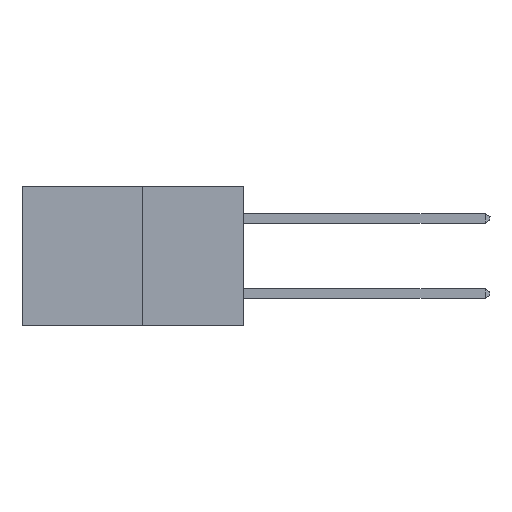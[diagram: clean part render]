
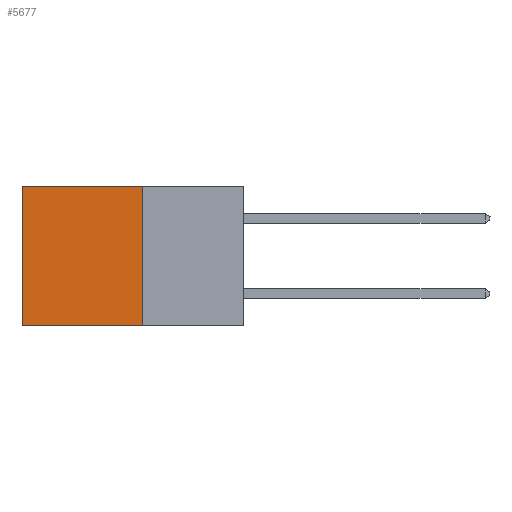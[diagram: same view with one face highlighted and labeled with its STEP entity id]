
A CAD part, left-side view. The second image highlights one B-rep face of the part: STEP entity #5677.
In plain terms, the highlighted planar face has unit normal (-1, 0, 0).
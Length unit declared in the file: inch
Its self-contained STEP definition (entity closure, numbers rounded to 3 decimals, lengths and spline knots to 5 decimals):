
#43 = ORIENTED_EDGE ( 'NONE', *, *, #1094, .T. ) ;
#718 = ORIENTED_EDGE ( 'NONE', *, *, #7204, .F. ) ;
#1094 = EDGE_CURVE ( 'NONE', #8426, #3668, #2150, .T. ) ;
#1461 = EDGE_CURVE ( 'NONE', #3668, #2317, #6913, .T. ) ;
#1546 = VECTOR ( 'NONE', #2091, 39.37008 ) ;
#1614 = CARTESIAN_POINT ( 'NONE',  ( 0.277, 0.27, -0.37 ) ) ;
#1648 = DIRECTION ( 'NONE',  ( 0., 1., 0. ) ) ;
#1667 = ORIENTED_EDGE ( 'NONE', *, *, #1461, .T. ) ;
#1909 = ORIENTED_EDGE ( 'NONE', *, *, #2686, .F. ) ;
#2091 = DIRECTION ( 'NONE',  ( 0., 1., 0. ) ) ;
#2150 = LINE ( 'NONE', #7919, #7536 ) ;
#2317 = VERTEX_POINT ( 'NONE', #6394 ) ;
#2346 = VERTEX_POINT ( 'NONE', #6817 ) ;
#2375 = DIRECTION ( 'NONE',  ( 0., 0., -1. ) ) ;
#2686 = EDGE_CURVE ( 'NONE', #2346, #2317, #3247, .T. ) ;
#2701 = FACE_OUTER_BOUND ( 'NONE', #6406, .T. ) ;
#3247 = LINE ( 'NONE', #8057, #1546 ) ;
#3306 = DIRECTION ( 'NONE',  ( 0., 0., -1. ) ) ;
#3668 = VERTEX_POINT ( 'NONE', #8718 ) ;
#4001 = CARTESIAN_POINT ( 'NONE',  ( 0.277, 0.27, -0.37 ) ) ;
#4382 = VECTOR ( 'NONE', #3306, 39.37008 ) ;
#5089 = PLANE ( 'NONE',  #7121 ) ;
#5159 = VECTOR ( 'NONE', #8526, 39.37008 ) ;
#5677 = ADVANCED_FACE ( 'NONE', ( #2701 ), #5089, .F. ) ;
#6394 = CARTESIAN_POINT ( 'NONE',  ( 0.277, 0.59, -0.37 ) ) ;
#6406 = EDGE_LOOP ( 'NONE', ( #1667, #1909, #718, #43 ) ) ;
#6429 = DIRECTION ( 'NONE',  ( 1., 0., 0. ) ) ;
#6817 = CARTESIAN_POINT ( 'NONE',  ( 0.277, 0.27, -0.37 ) ) ;
#6913 = LINE ( 'NONE', #8594, #5159 ) ;
#7121 = AXIS2_PLACEMENT_3D ( 'NONE', #1614, #6429, #2375 ) ;
#7204 = EDGE_CURVE ( 'NONE', #8426, #2346, #7926, .T. ) ;
#7536 = VECTOR ( 'NONE', #1648, 39.37008 ) ;
#7919 = CARTESIAN_POINT ( 'NONE',  ( 0.277, 0.27, 0. ) ) ;
#7926 = LINE ( 'NONE', #4001, #4382 ) ;
#8057 = CARTESIAN_POINT ( 'NONE',  ( 0.277, 0.27, -0.37 ) ) ;
#8371 = CARTESIAN_POINT ( 'NONE',  ( 0.277, 0.27, 0. ) ) ;
#8426 = VERTEX_POINT ( 'NONE', #8371 ) ;
#8526 = DIRECTION ( 'NONE',  ( 0., 0., -1. ) ) ;
#8594 = CARTESIAN_POINT ( 'NONE',  ( 0.277, 0.59, -0.37 ) ) ;
#8718 = CARTESIAN_POINT ( 'NONE',  ( 0.277, 0.59, 0. ) ) ;
